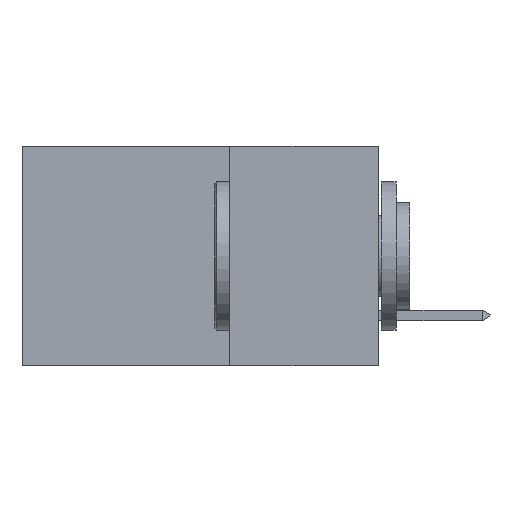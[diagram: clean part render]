
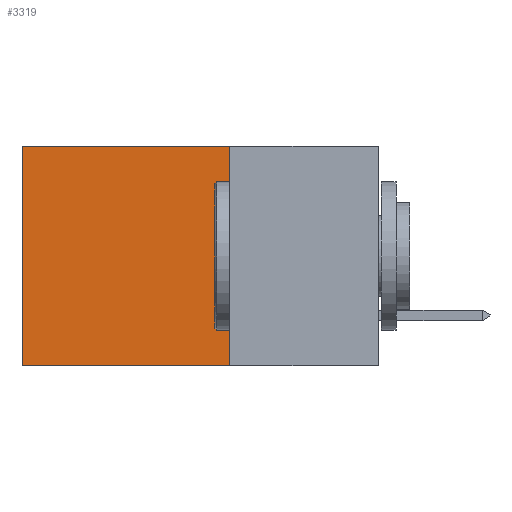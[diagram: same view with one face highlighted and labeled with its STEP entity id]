
A CAD part, left-side view. The second image highlights one B-rep face of the part: STEP entity #3319.
In plain terms, the highlighted planar face has unit normal (-1, 0, 0).
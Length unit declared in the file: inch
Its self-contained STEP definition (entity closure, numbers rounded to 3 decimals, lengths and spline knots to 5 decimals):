
#49 = CARTESIAN_POINT ( 'NONE',  ( 0.2615, 0.25, -0.37 ) ) ;
#107 = FACE_OUTER_BOUND ( 'NONE', #3590, .T. ) ;
#437 = DIRECTION ( 'NONE',  ( 0., 0., -1. ) ) ;
#1030 = CARTESIAN_POINT ( 'NONE',  ( 0.2615, 0.25, -0.37 ) ) ;
#1205 = DIRECTION ( 'NONE',  ( 0., 1., 0. ) ) ;
#1225 = LINE ( 'NONE', #10206, #9166 ) ;
#1760 = VECTOR ( 'NONE', #6204, 39.37008 ) ;
#2345 = ORIENTED_EDGE ( 'NONE', *, *, #10726, .T. ) ;
#2360 = CARTESIAN_POINT ( 'NONE',  ( 0.2615, 0.6, -0.37 ) ) ;
#2432 = CARTESIAN_POINT ( 'NONE',  ( 0.2615, 0.6, -0.37 ) ) ;
#2557 = EDGE_CURVE ( 'NONE', #6614, #10584, #1225, .T. ) ;
#2772 = LINE ( 'NONE', #1030, #4875 ) ;
#3319 = ADVANCED_FACE ( 'NONE', ( #107 ), #6160, .F. ) ;
#3347 = LINE ( 'NONE', #6919, #1760 ) ;
#3530 = EDGE_CURVE ( 'NONE', #6614, #10022, #3347, .T. ) ;
#3590 = EDGE_LOOP ( 'NONE', ( #2345, #10792, #9473, #10850 ) ) ;
#4768 = VERTEX_POINT ( 'NONE', #2432 ) ;
#4875 = VECTOR ( 'NONE', #1205, 39.37008 ) ;
#5469 = AXIS2_PLACEMENT_3D ( 'NONE', #49, #8850, #7496 ) ;
#6160 = PLANE ( 'NONE',  #5469 ) ;
#6204 = DIRECTION ( 'NONE',  ( 0., 0., -1. ) ) ;
#6362 = CARTESIAN_POINT ( 'NONE',  ( 0.2615, 0.6, 0. ) ) ;
#6614 = VERTEX_POINT ( 'NONE', #11232 ) ;
#6919 = CARTESIAN_POINT ( 'NONE',  ( 0.2615, 0.25, -0.37 ) ) ;
#7233 = EDGE_CURVE ( 'NONE', #10022, #4768, #2772, .T. ) ;
#7242 = DIRECTION ( 'NONE',  ( 0., 1., 0. ) ) ;
#7496 = DIRECTION ( 'NONE',  ( 0., 0., -1. ) ) ;
#7500 = VECTOR ( 'NONE', #437, 39.37008 ) ;
#7788 = CARTESIAN_POINT ( 'NONE',  ( 0.2615, 0.25, -0.37 ) ) ;
#8850 = DIRECTION ( 'NONE',  ( 1., 0., 0. ) ) ;
#9166 = VECTOR ( 'NONE', #7242, 39.37008 ) ;
#9363 = LINE ( 'NONE', #2360, #7500 ) ;
#9473 = ORIENTED_EDGE ( 'NONE', *, *, #3530, .F. ) ;
#10022 = VERTEX_POINT ( 'NONE', #7788 ) ;
#10206 = CARTESIAN_POINT ( 'NONE',  ( 0.2615, 0.25, 0. ) ) ;
#10584 = VERTEX_POINT ( 'NONE', #6362 ) ;
#10726 = EDGE_CURVE ( 'NONE', #10584, #4768, #9363, .T. ) ;
#10792 = ORIENTED_EDGE ( 'NONE', *, *, #7233, .F. ) ;
#10850 = ORIENTED_EDGE ( 'NONE', *, *, #2557, .T. ) ;
#11232 = CARTESIAN_POINT ( 'NONE',  ( 0.2615, 0.25, 0. ) ) ;
